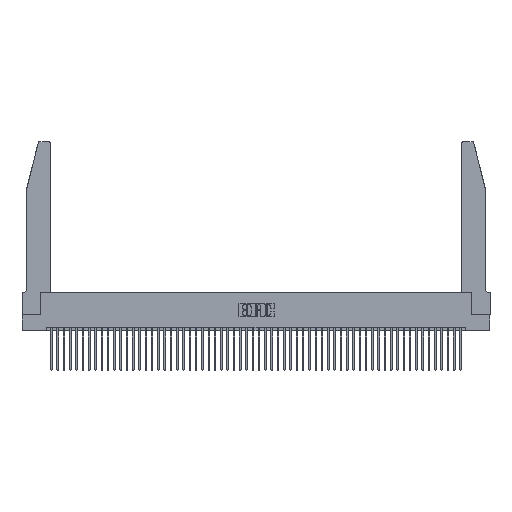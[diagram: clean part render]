
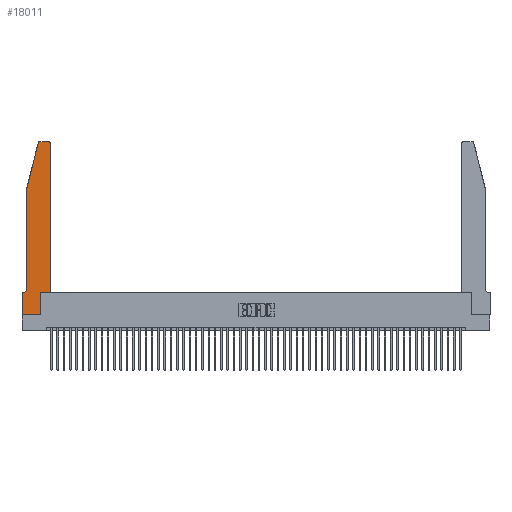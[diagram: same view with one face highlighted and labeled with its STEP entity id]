
A CAD part, top view. The second image highlights one B-rep face of the part: STEP entity #18011.
In plain terms, the highlighted planar face has unit normal (0, 0, 1).
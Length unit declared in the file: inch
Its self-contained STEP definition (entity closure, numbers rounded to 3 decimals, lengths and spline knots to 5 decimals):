
#180 = LINE ( 'NONE', #15922, #18844 ) ;
#310 = EDGE_CURVE ( 'NONE', #42547, #33457, #29398, .T. ) ;
#1984 = ORIENTED_EDGE ( 'NONE', *, *, #21569, .T. ) ;
#2233 = VERTEX_POINT ( 'NONE', #38535 ) ;
#2285 = DIRECTION ( 'NONE',  ( 0., 1., 0. ) ) ;
#2867 = DIRECTION ( 'NONE',  ( 1., 0., 0. ) ) ;
#3001 = DIRECTION ( 'NONE',  ( 0., -1., 0. ) ) ;
#3191 = DIRECTION ( 'NONE',  ( 1., 0., 0. ) ) ;
#3871 = ORIENTED_EDGE ( 'NONE', *, *, #38519, .T. ) ;
#4946 = CARTESIAN_POINT ( 'NONE',  ( 0.0055, 0.42, 0.37 ) ) ;
#5107 = LINE ( 'NONE', #19907, #26346 ) ;
#5277 = FACE_OUTER_BOUND ( 'NONE', #14248, .T. ) ;
#5512 = CARTESIAN_POINT ( 'NONE',  ( 0.2865, 0.35, 0.37 ) ) ;
#5572 = CARTESIAN_POINT ( 'NONE',  ( 0.0055, 0.35, 0.37 ) ) ;
#5929 = VERTEX_POINT ( 'NONE', #47363 ) ;
#7367 = EDGE_CURVE ( 'NONE', #33457, #2233, #36067, .T. ) ;
#7495 = CARTESIAN_POINT ( 'NONE',  ( 0.0755, 0.35, 0.37 ) ) ;
#8371 = DIRECTION ( 'NONE',  ( 1., 0., 0. ) ) ;
#8401 = CARTESIAN_POINT ( 'NONE',  ( 0.2605, 2.75, 0.37 ) ) ;
#9726 = ORIENTED_EDGE ( 'NONE', *, *, #37069, .T. ) ;
#10472 = ORIENTED_EDGE ( 'NONE', *, *, #44056, .T. ) ;
#10630 = ORIENTED_EDGE ( 'NONE', *, *, #310, .T. ) ;
#10730 = VERTEX_POINT ( 'NONE', #47442 ) ;
#10819 = CARTESIAN_POINT ( 'NONE',  ( 0.0755, 2., 0.37 ) ) ;
#11414 = CARTESIAN_POINT ( 'NONE',  ( 0.0755, 2., 0.37 ) ) ;
#13122 = DIRECTION ( 'NONE',  ( 0., -1., 0. ) ) ;
#14015 = AXIS2_PLACEMENT_3D ( 'NONE', #47704, #47526, #39543 ) ;
#14248 = EDGE_LOOP ( 'NONE', ( #28232, #41528, #23261, #36161, #34892, #1984, #41889, #9726, #3871, #26429, #10472, #10630 ) ) ;
#14696 = VERTEX_POINT ( 'NONE', #5572 ) ;
#15433 = VECTOR ( 'NONE', #45384, 39.37008 ) ;
#15482 = AXIS2_PLACEMENT_3D ( 'NONE', #33373, #21220, #50042 ) ;
#15922 = CARTESIAN_POINT ( 'NONE',  ( 0., 0., 0.37 ) ) ;
#16454 = DIRECTION ( 'NONE',  ( -1., 0., 0. ) ) ;
#16537 = CARTESIAN_POINT ( 'NONE',  ( 0.2865, 0.35, 0.37 ) ) ;
#18011 = ADVANCED_FACE ( 'NONE', ( #5277 ), #44439, .T. ) ;
#18712 = LINE ( 'NONE', #7495, #37408 ) ;
#18844 = VECTOR ( 'NONE', #3001, 39.37008 ) ;
#19907 = CARTESIAN_POINT ( 'NONE',  ( 0.4505, 0.35, 0.37 ) ) ;
#20833 = DIRECTION ( 'NONE',  ( -1., 0., 0. ) ) ;
#21220 = DIRECTION ( 'NONE',  ( 0., 0., 1. ) ) ;
#21528 = LINE ( 'NONE', #30518, #22139 ) ;
#21569 = EDGE_CURVE ( 'NONE', #14696, #38610, #18712, .T. ) ;
#21729 = VERTEX_POINT ( 'NONE', #28881 ) ;
#21940 = LINE ( 'NONE', #16537, #15433 ) ;
#21957 = VECTOR ( 'NONE', #20833, 39.37008 ) ;
#22139 = VECTOR ( 'NONE', #2285, 39.37008 ) ;
#23261 = ORIENTED_EDGE ( 'NONE', *, *, #37554, .T. ) ;
#23368 = VERTEX_POINT ( 'NONE', #47741 ) ;
#23563 = CIRCLE ( 'NONE', #42787, 0.07 ) ;
#23957 = LINE ( 'NONE', #10819, #44571 ) ;
#24284 = CARTESIAN_POINT ( 'NONE',  ( 0.25487, 2.72718, 0.37 ) ) ;
#25470 = CARTESIAN_POINT ( 'NONE',  ( 0.4205, 2.75, 0.37 ) ) ;
#25945 = CARTESIAN_POINT ( 'NONE',  ( 0.0755, 2., 0.37 ) ) ;
#25959 = VECTOR ( 'NONE', #8371, 39.37008 ) ;
#26346 = VECTOR ( 'NONE', #3191, 39.37008 ) ;
#26429 = ORIENTED_EDGE ( 'NONE', *, *, #49618, .T. ) ;
#27860 = CARTESIAN_POINT ( 'NONE',  ( 0., 0.35, 0.37 ) ) ;
#28232 = ORIENTED_EDGE ( 'NONE', *, *, #7367, .T. ) ;
#28851 = CARTESIAN_POINT ( 'NONE',  ( 0.4505, 2.72, 0.37 ) ) ;
#28881 = CARTESIAN_POINT ( 'NONE',  ( 0.2865, 0., 0.37 ) ) ;
#29173 = EDGE_CURVE ( 'NONE', #2233, #34552, #50211, .T. ) ;
#29274 = VERTEX_POINT ( 'NONE', #11414 ) ;
#29398 = CIRCLE ( 'NONE', #15482, 0.03 ) ;
#30518 = CARTESIAN_POINT ( 'NONE',  ( 0.4505, 0.35, 0.37 ) ) ;
#31393 = EDGE_CURVE ( 'NONE', #5929, #14696, #23563, .T. ) ;
#33054 = VERTEX_POINT ( 'NONE', #5512 ) ;
#33373 = CARTESIAN_POINT ( 'NONE',  ( 0.4205, 2.72, 0.37 ) ) ;
#33457 = VERTEX_POINT ( 'NONE', #25470 ) ;
#33876 = DIRECTION ( 'NONE',  ( -1., 0., 0. ) ) ;
#34275 = EDGE_CURVE ( 'NONE', #29274, #5929, #34585, .T. ) ;
#34552 = VERTEX_POINT ( 'NONE', #24284 ) ;
#34585 = LINE ( 'NONE', #25945, #44978 ) ;
#34892 = ORIENTED_EDGE ( 'NONE', *, *, #31393, .T. ) ;
#36067 = LINE ( 'NONE', #8401, #21957 ) ;
#36161 = ORIENTED_EDGE ( 'NONE', *, *, #34275, .T. ) ;
#37011 = EDGE_CURVE ( 'NONE', #38610, #10730, #180, .T. ) ;
#37069 = EDGE_CURVE ( 'NONE', #10730, #21729, #42722, .T. ) ;
#37408 = VECTOR ( 'NONE', #16454, 39.37008 ) ;
#37554 = EDGE_CURVE ( 'NONE', #34552, #29274, #23957, .T. ) ;
#38519 = EDGE_CURVE ( 'NONE', #21729, #33054, #21940, .T. ) ;
#38535 = CARTESIAN_POINT ( 'NONE',  ( 0.284, 2.75, 0.37 ) ) ;
#38610 = VERTEX_POINT ( 'NONE', #42674 ) ;
#38945 = AXIS2_PLACEMENT_3D ( 'NONE', #27860, #39944, #2867 ) ;
#39543 = DIRECTION ( 'NONE',  ( 1., 0., 0. ) ) ;
#39944 = DIRECTION ( 'NONE',  ( 0., 0., 1. ) ) ;
#41528 = ORIENTED_EDGE ( 'NONE', *, *, #29173, .T. ) ;
#41889 = ORIENTED_EDGE ( 'NONE', *, *, #37011, .T. ) ;
#42547 = VERTEX_POINT ( 'NONE', #28851 ) ;
#42674 = CARTESIAN_POINT ( 'NONE',  ( 0., 0.35, 0.37 ) ) ;
#42722 = LINE ( 'NONE', #48240, #25959 ) ;
#42787 = AXIS2_PLACEMENT_3D ( 'NONE', #4946, #50192, #33876 ) ;
#44056 = EDGE_CURVE ( 'NONE', #23368, #42547, #21528, .T. ) ;
#44439 = PLANE ( 'NONE',  #38945 ) ;
#44571 = VECTOR ( 'NONE', #51591, 39.37008 ) ;
#44978 = VECTOR ( 'NONE', #13122, 39.37008 ) ;
#45384 = DIRECTION ( 'NONE',  ( 0., 1., 0. ) ) ;
#47363 = CARTESIAN_POINT ( 'NONE',  ( 0.0755, 0.42, 0.37 ) ) ;
#47442 = CARTESIAN_POINT ( 'NONE',  ( 0., 0., 0.37 ) ) ;
#47526 = DIRECTION ( 'NONE',  ( 0., 0., 1. ) ) ;
#47704 = CARTESIAN_POINT ( 'NONE',  ( 0.284, 2.72, 0.37 ) ) ;
#47741 = CARTESIAN_POINT ( 'NONE',  ( 0.4505, 0.35, 0.37 ) ) ;
#48240 = CARTESIAN_POINT ( 'NONE',  ( 0., 0., 0.37 ) ) ;
#49618 = EDGE_CURVE ( 'NONE', #33054, #23368, #5107, .T. ) ;
#50042 = DIRECTION ( 'NONE',  ( 1., 0., 0. ) ) ;
#50192 = DIRECTION ( 'NONE',  ( 0., 0., -1. ) ) ;
#50211 = CIRCLE ( 'NONE', #14015, 0.03 ) ;
#51591 = DIRECTION ( 'NONE',  ( -0.239, -0.971, 0. ) ) ;
